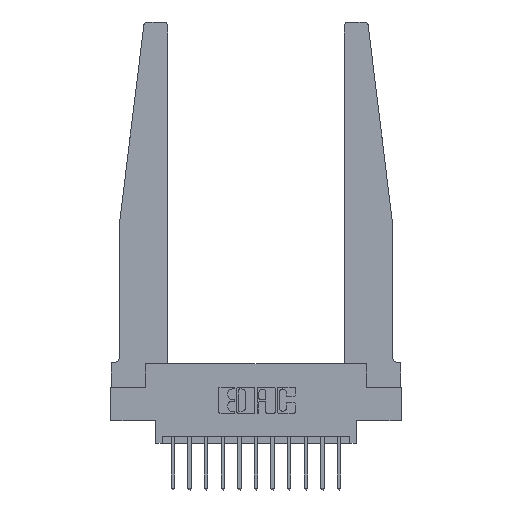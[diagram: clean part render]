
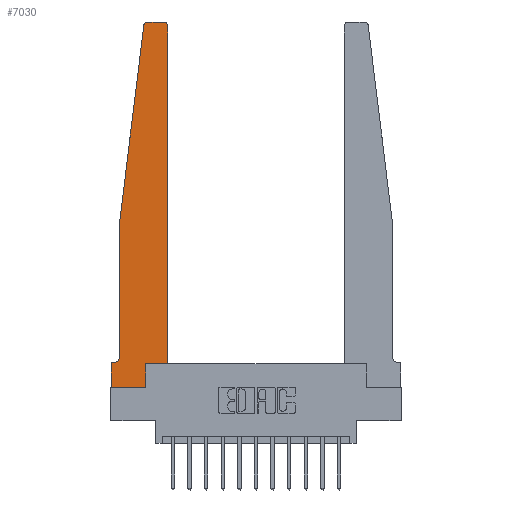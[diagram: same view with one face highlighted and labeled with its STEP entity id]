
A CAD part, top view. The second image highlights one B-rep face of the part: STEP entity #7030.
In plain terms, the highlighted planar face has unit normal (0, 0, 1).
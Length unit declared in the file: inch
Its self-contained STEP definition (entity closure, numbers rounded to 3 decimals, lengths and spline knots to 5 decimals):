
#177 = EDGE_CURVE ( 'NONE', #12240, #8257, #5301, .T. ) ;
#295 = DIRECTION ( 'NONE',  ( 0., -1., 0. ) ) ;
#415 = LINE ( 'NONE', #16031, #9690 ) ;
#500 = VECTOR ( 'NONE', #295, 39.37008 ) ;
#620 = DIRECTION ( 'NONE',  ( 1., 0., 0. ) ) ;
#648 = VECTOR ( 'NONE', #3226, 39.37008 ) ;
#970 = FACE_OUTER_BOUND ( 'NONE', #5525, .T. ) ;
#1070 = DIRECTION ( 'NONE',  ( 0., 1., 0. ) ) ;
#1101 = CARTESIAN_POINT ( 'NONE',  ( 0.065, 0.2375, 0.37 ) ) ;
#1418 = CARTESIAN_POINT ( 'NONE',  ( 0.015, 0.2375, 0.37 ) ) ;
#1569 = CARTESIAN_POINT ( 'NONE',  ( 0.015, 0.1875, 0.37 ) ) ;
#1690 = CARTESIAN_POINT ( 'NONE',  ( 0., 0., 0.37 ) ) ;
#1758 = VERTEX_POINT ( 'NONE', #8363 ) ;
#1778 = EDGE_CURVE ( 'NONE', #2275, #12240, #415, .T. ) ;
#2139 = CARTESIAN_POINT ( 'NONE',  ( 0.425, 0.18, 0.37 ) ) ;
#2267 = ORIENTED_EDGE ( 'NONE', *, *, #4906, .T. ) ;
#2275 = VERTEX_POINT ( 'NONE', #6268 ) ;
#2279 = DIRECTION ( 'NONE',  ( 1., 0., 0. ) ) ;
#2858 = CIRCLE ( 'NONE', #10199, 0.03 ) ;
#3096 = LINE ( 'NONE', #12353, #9699 ) ;
#3226 = DIRECTION ( 'NONE',  ( -1., 0., 0. ) ) ;
#3316 = DIRECTION ( 'NONE',  ( 1., 0., 0. ) ) ;
#3378 = LINE ( 'NONE', #11221, #7761 ) ;
#3576 = VERTEX_POINT ( 'NONE', #8451 ) ;
#3584 = ORIENTED_EDGE ( 'NONE', *, *, #7841, .T. ) ;
#3850 = VECTOR ( 'NONE', #1070, 39.37008 ) ;
#4228 = ORIENTED_EDGE ( 'NONE', *, *, #7571, .T. ) ;
#4327 = EDGE_CURVE ( 'NONE', #15954, #2275, #2858, .T. ) ;
#4598 = ORIENTED_EDGE ( 'NONE', *, *, #177, .T. ) ;
#4880 = DIRECTION ( 'NONE',  ( 0., 0., 1. ) ) ;
#4906 = EDGE_CURVE ( 'NONE', #14370, #11902, #16096, .T. ) ;
#4919 = CARTESIAN_POINT ( 'NONE',  ( 0.2605, 0.18, 0.37 ) ) ;
#5080 = CARTESIAN_POINT ( 'NONE',  ( 0.065, 1.25, 0.37 ) ) ;
#5082 = DIRECTION ( 'NONE',  ( 0., 0., 1. ) ) ;
#5301 = LINE ( 'NONE', #10491, #500 ) ;
#5321 = ORIENTED_EDGE ( 'NONE', *, *, #4327, .T. ) ;
#5525 = EDGE_LOOP ( 'NONE', ( #3584, #5321, #6942, #4598, #6529, #5747, #14770, #4228, #5668, #6632, #12815, #2267 ) ) ;
#5546 = CARTESIAN_POINT ( 'NONE',  ( 0.395, 2.72, 0.37 ) ) ;
#5668 = ORIENTED_EDGE ( 'NONE', *, *, #5770, .T. ) ;
#5747 = ORIENTED_EDGE ( 'NONE', *, *, #14872, .T. ) ;
#5770 = EDGE_CURVE ( 'NONE', #3576, #6037, #3378, .T. ) ;
#5942 = CARTESIAN_POINT ( 'NONE',  ( 0.425, 0.18, 0.37 ) ) ;
#6037 = VERTEX_POINT ( 'NONE', #4919 ) ;
#6135 = PLANE ( 'NONE',  #10140 ) ;
#6268 = CARTESIAN_POINT ( 'NONE',  ( 0.24675, 2.72367, 0.37 ) ) ;
#6523 = LINE ( 'NONE', #8934, #16151 ) ;
#6529 = ORIENTED_EDGE ( 'NONE', *, *, #12100, .T. ) ;
#6580 = DIRECTION ( 'NONE',  ( -1., 0., 0. ) ) ;
#6632 = ORIENTED_EDGE ( 'NONE', *, *, #10742, .T. ) ;
#6881 = DIRECTION ( 'NONE',  ( 1., 0., 0. ) ) ;
#6942 = ORIENTED_EDGE ( 'NONE', *, *, #1778, .T. ) ;
#7030 = ADVANCED_FACE ( 'NONE', ( #970 ), #6135, .T. ) ;
#7571 = EDGE_CURVE ( 'NONE', #1758, #3576, #13320, .T. ) ;
#7581 = CARTESIAN_POINT ( 'NONE',  ( 0.27653, 2.75, 0.37 ) ) ;
#7592 = DIRECTION ( 'NONE',  ( 0., -1., 0. ) ) ;
#7761 = VECTOR ( 'NONE', #15065, 39.37008 ) ;
#7841 = EDGE_CURVE ( 'NONE', #11902, #15954, #16261, .T. ) ;
#7993 = VERTEX_POINT ( 'NONE', #10962 ) ;
#8257 = VERTEX_POINT ( 'NONE', #1101 ) ;
#8363 = CARTESIAN_POINT ( 'NONE',  ( 0., 0., 0.37 ) ) ;
#8432 = AXIS2_PLACEMENT_3D ( 'NONE', #1418, #15457, #6580 ) ;
#8451 = CARTESIAN_POINT ( 'NONE',  ( 0.2605, 0., 0.37 ) ) ;
#8663 = VERTEX_POINT ( 'NONE', #13858 ) ;
#8784 = CARTESIAN_POINT ( 'NONE',  ( 0., 0.1875, 0.37 ) ) ;
#8934 = CARTESIAN_POINT ( 'NONE',  ( 0.065, 0.1875, 0.37 ) ) ;
#9219 = CARTESIAN_POINT ( 'NONE',  ( 0.27653, 2.72, 0.37 ) ) ;
#9393 = VERTEX_POINT ( 'NONE', #1569 ) ;
#9690 = VECTOR ( 'NONE', #10785, 39.37008 ) ;
#9699 = VECTOR ( 'NONE', #7592, 39.37008 ) ;
#9986 = EDGE_CURVE ( 'NONE', #8663, #14370, #15260, .T. ) ;
#10140 = AXIS2_PLACEMENT_3D ( 'NONE', #8784, #4880, #3316 ) ;
#10199 = AXIS2_PLACEMENT_3D ( 'NONE', #9219, #5082, #11538 ) ;
#10491 = CARTESIAN_POINT ( 'NONE',  ( 0.065, 1.25, 0.37 ) ) ;
#10742 = EDGE_CURVE ( 'NONE', #6037, #8663, #11289, .T. ) ;
#10785 = DIRECTION ( 'NONE',  ( -0.122, -0.992, 0. ) ) ;
#10962 = CARTESIAN_POINT ( 'NONE',  ( 0., 0.1875, 0.37 ) ) ;
#11221 = CARTESIAN_POINT ( 'NONE',  ( 0.2605, 0.18, 0.37 ) ) ;
#11289 = LINE ( 'NONE', #5942, #12229 ) ;
#11538 = DIRECTION ( 'NONE',  ( 1., 0., 0. ) ) ;
#11734 = CIRCLE ( 'NONE', #8432, 0.05 ) ;
#11902 = VERTEX_POINT ( 'NONE', #16208 ) ;
#12100 = EDGE_CURVE ( 'NONE', #8257, #9393, #11734, .T. ) ;
#12229 = VECTOR ( 'NONE', #2279, 39.37008 ) ;
#12240 = VERTEX_POINT ( 'NONE', #5080 ) ;
#12241 = DIRECTION ( 'NONE',  ( 0., 0., 1. ) ) ;
#12353 = CARTESIAN_POINT ( 'NONE',  ( 0., 0., 0.37 ) ) ;
#12815 = ORIENTED_EDGE ( 'NONE', *, *, #9986, .T. ) ;
#13320 = LINE ( 'NONE', #1690, #15778 ) ;
#13357 = CARTESIAN_POINT ( 'NONE',  ( 0.425, 2.72, 0.37 ) ) ;
#13651 = EDGE_CURVE ( 'NONE', #7993, #1758, #3096, .T. ) ;
#13858 = CARTESIAN_POINT ( 'NONE',  ( 0.425, 0.18, 0.37 ) ) ;
#14370 = VERTEX_POINT ( 'NONE', #13357 ) ;
#14770 = ORIENTED_EDGE ( 'NONE', *, *, #13651, .T. ) ;
#14848 = CARTESIAN_POINT ( 'NONE',  ( 0.25, 2.75, 0.37 ) ) ;
#14872 = EDGE_CURVE ( 'NONE', #9393, #7993, #6523, .T. ) ;
#15065 = DIRECTION ( 'NONE',  ( 0., 1., 0. ) ) ;
#15260 = LINE ( 'NONE', #2139, #3850 ) ;
#15457 = DIRECTION ( 'NONE',  ( 0., 0., -1. ) ) ;
#15578 = AXIS2_PLACEMENT_3D ( 'NONE', #5546, #12241, #620 ) ;
#15778 = VECTOR ( 'NONE', #6881, 39.37008 ) ;
#15954 = VERTEX_POINT ( 'NONE', #7581 ) ;
#16031 = CARTESIAN_POINT ( 'NONE',  ( 0.065, 1.25, 0.37 ) ) ;
#16096 = CIRCLE ( 'NONE', #15578, 0.03 ) ;
#16151 = VECTOR ( 'NONE', #16670, 39.37008 ) ;
#16208 = CARTESIAN_POINT ( 'NONE',  ( 0.395, 2.75, 0.37 ) ) ;
#16261 = LINE ( 'NONE', #14848, #648 ) ;
#16670 = DIRECTION ( 'NONE',  ( -1., 0., 0. ) ) ;
